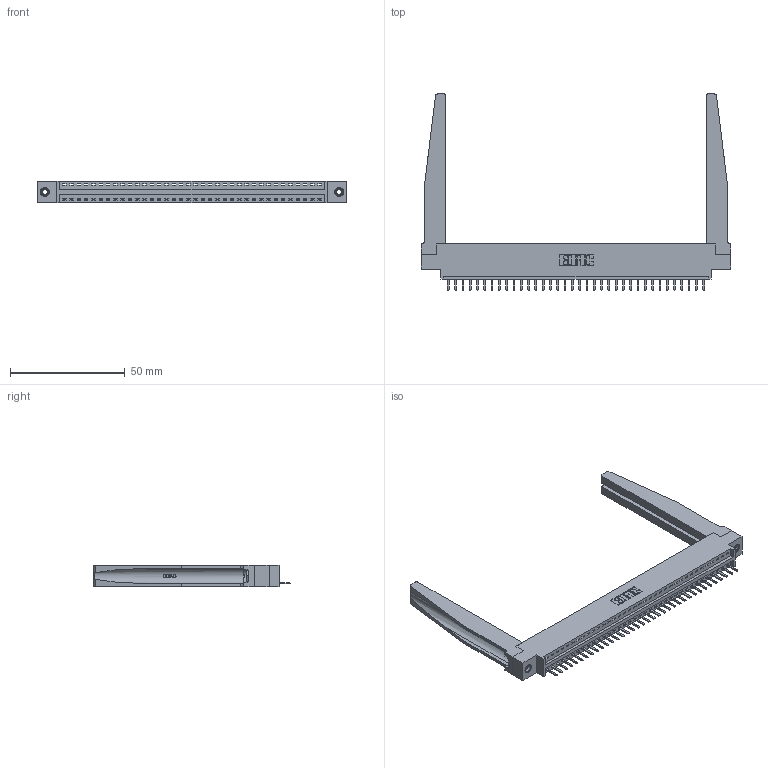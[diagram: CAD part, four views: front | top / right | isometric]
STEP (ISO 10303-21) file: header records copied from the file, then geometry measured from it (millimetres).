
FILE_DESCRIPTION (( 'STEP AP203' ), '1' );
FILE_NAME ('346-036-520-678.STEP', '2022-05-07T00:24:42', ( '' ), ( '' ), 'SwSTEP 2.0', 'SolidWorks 2020', '' );
FILE_SCHEMA (( 'CONFIG_CONTROL_DESIGN' ));
Length unit declared in the file: inch
Products named in the file (5): 346-220-078_345-220-078; 346 Part_0.170 Offset - 0.156 Dia-TH; 345-292-001_345-293-120; 345-250-001_345-250-001-102; 346-036-520-678
Assembly tree (41 placements, depth 2):
  346-036-520-678
    346 Part_0.170 Offset - 0.156 Dia-TH
    345-292-001_345-293-120  x36
    346-220-078_345-220-078  x2
    345-250-001_345-250-001-102  x2
Bounding box: 134.87 x 85.29 x 9.4 mm (x, y, z)
Volume: 19501.7 mm3; surface area: 22061.7 mm2
Topology: 41 solids, 41 shells, 2606 faces, 7609 edges, 4966 vertices
Faces by surface type: plane 1748, cylinder 806, bspline 36, cone 12, torus 4
Entity records: 28560 total; most frequent: CARTESIAN_POINT 5825, ORIENTED_EDGE 4670, DIRECTION 4117, EDGE_CURVE 2335, VECTOR 1961, LINE 1961, VERTEX_POINT 1548, AXIS2_PLACEMENT_3D 1078
